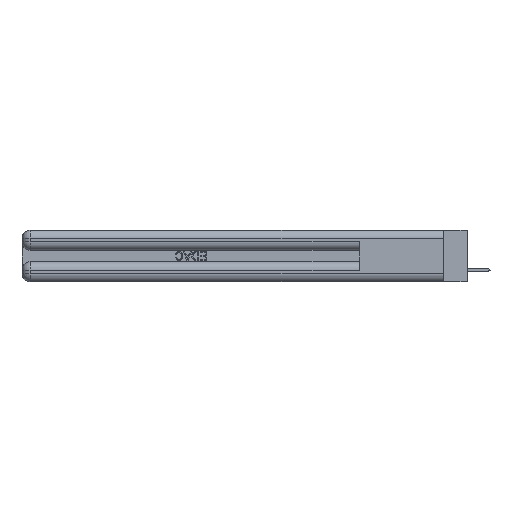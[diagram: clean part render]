
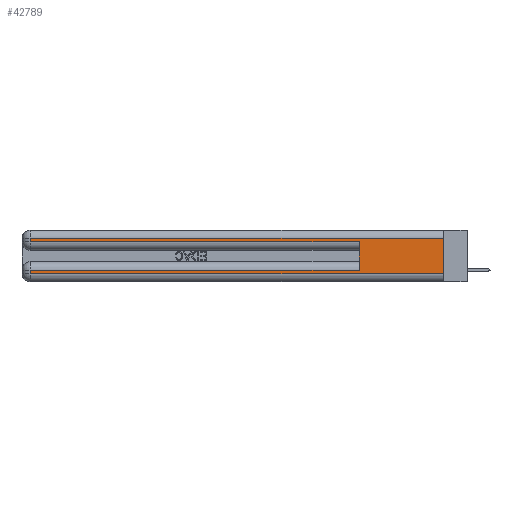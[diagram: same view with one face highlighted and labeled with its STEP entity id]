
A CAD part, left-side view. The second image highlights one B-rep face of the part: STEP entity #42789.
In plain terms, the highlighted planar face has unit normal (-1, 0, 0).
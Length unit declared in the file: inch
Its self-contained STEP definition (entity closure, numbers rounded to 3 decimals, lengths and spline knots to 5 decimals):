
#2408 = EDGE_CURVE ( 'NONE', #15796, #23937, #38843, .T. ) ;
#2837 = CARTESIAN_POINT ( 'NONE',  ( 0., 0., 0.31 ) ) ;
#3626 = DIRECTION ( 'NONE',  ( 0., 0., -1. ) ) ;
#3765 = LINE ( 'NONE', #13259, #15611 ) ;
#5084 = CARTESIAN_POINT ( 'NONE',  ( 0., 0., 0.285 ) ) ;
#5658 = LINE ( 'NONE', #5084, #23727 ) ;
#5894 = ORIENTED_EDGE ( 'NONE', *, *, #13150, .F. ) ;
#7551 = LINE ( 'NONE', #28737, #14400 ) ;
#7577 = LINE ( 'NONE', #15505, #40936 ) ;
#8554 = CARTESIAN_POINT ( 'NONE',  ( 0., 0., 0.085 ) ) ;
#9575 = ORIENTED_EDGE ( 'NONE', *, *, #38230, .T. ) ;
#9879 = EDGE_CURVE ( 'NONE', #10290, #16797, #5658, .T. ) ;
#10290 = VERTEX_POINT ( 'NONE', #37390 ) ;
#11018 = DIRECTION ( 'NONE',  ( 0., 1., 0. ) ) ;
#11537 = VECTOR ( 'NONE', #33886, 39.37008 ) ;
#12793 = CARTESIAN_POINT ( 'NONE',  ( 0., 0.6, 0.085 ) ) ;
#13150 = EDGE_CURVE ( 'NONE', #23504, #21130, #26059, .T. ) ;
#13259 = CARTESIAN_POINT ( 'NONE',  ( 0., 0., 0.06 ) ) ;
#14400 = VECTOR ( 'NONE', #11018, 39.37008 ) ;
#15348 = CARTESIAN_POINT ( 'NONE',  ( 0., 0., 0.37 ) ) ;
#15505 = CARTESIAN_POINT ( 'NONE',  ( 0., 0.6, 0.145 ) ) ;
#15611 = VECTOR ( 'NONE', #27459, 39.37008 ) ;
#15796 = VERTEX_POINT ( 'NONE', #34582 ) ;
#15822 = ORIENTED_EDGE ( 'NONE', *, *, #44929, .T. ) ;
#16546 = ORIENTED_EDGE ( 'NONE', *, *, #31710, .T. ) ;
#16797 = VERTEX_POINT ( 'NONE', #38414 ) ;
#17389 = CARTESIAN_POINT ( 'NONE',  ( 0., 2.94, 0.06 ) ) ;
#19365 = CARTESIAN_POINT ( 'NONE',  ( 0., 0., 0.37 ) ) ;
#19902 = EDGE_CURVE ( 'NONE', #32968, #16797, #7577, .T. ) ;
#20515 = AXIS2_PLACEMENT_3D ( 'NONE', #15348, #44396, #40641 ) ;
#20776 = VERTEX_POINT ( 'NONE', #32190 ) ;
#21130 = VERTEX_POINT ( 'NONE', #23594 ) ;
#21826 = VECTOR ( 'NONE', #3626, 39.37008 ) ;
#22173 = DIRECTION ( 'NONE',  ( 0., -1., 0. ) ) ;
#23504 = VERTEX_POINT ( 'NONE', #2837 ) ;
#23594 = CARTESIAN_POINT ( 'NONE',  ( 0., 0., 0.06 ) ) ;
#23727 = VECTOR ( 'NONE', #22173, 39.37008 ) ;
#23937 = VERTEX_POINT ( 'NONE', #17389 ) ;
#25581 = CARTESIAN_POINT ( 'NONE',  ( 0., 2.94, 0.37 ) ) ;
#26059 = LINE ( 'NONE', #19365, #28944 ) ;
#27459 = DIRECTION ( 'NONE',  ( 0., -1., 0. ) ) ;
#28737 = CARTESIAN_POINT ( 'NONE',  ( 0., 0., 0.31 ) ) ;
#28944 = VECTOR ( 'NONE', #34792, 39.37008 ) ;
#29761 = PLANE ( 'NONE',  #20515 ) ;
#31118 = FACE_OUTER_BOUND ( 'NONE', #32379, .T. ) ;
#31710 = EDGE_CURVE ( 'NONE', #23504, #20776, #7551, .T. ) ;
#32190 = CARTESIAN_POINT ( 'NONE',  ( 0., 2.94, 0.31 ) ) ;
#32365 = LINE ( 'NONE', #35673, #33428 ) ;
#32379 = EDGE_LOOP ( 'NONE', ( #5894, #16546, #15822, #42070, #40188, #36386, #36863, #9575 ) ) ;
#32525 = LINE ( 'NONE', #8554, #11537 ) ;
#32968 = VERTEX_POINT ( 'NONE', #12793 ) ;
#33428 = VECTOR ( 'NONE', #46225, 39.37008 ) ;
#33886 = DIRECTION ( 'NONE',  ( 0., 1., 0. ) ) ;
#34582 = CARTESIAN_POINT ( 'NONE',  ( 0., 2.94, 0.085 ) ) ;
#34792 = DIRECTION ( 'NONE',  ( 0., 0., -1. ) ) ;
#35673 = CARTESIAN_POINT ( 'NONE',  ( 0., 2.94, 0.37 ) ) ;
#36386 = ORIENTED_EDGE ( 'NONE', *, *, #39720, .T. ) ;
#36863 = ORIENTED_EDGE ( 'NONE', *, *, #2408, .T. ) ;
#37390 = CARTESIAN_POINT ( 'NONE',  ( 0., 2.94, 0.285 ) ) ;
#38230 = EDGE_CURVE ( 'NONE', #23937, #21130, #3765, .T. ) ;
#38414 = CARTESIAN_POINT ( 'NONE',  ( 0., 0.6, 0.285 ) ) ;
#38843 = LINE ( 'NONE', #25581, #21826 ) ;
#39720 = EDGE_CURVE ( 'NONE', #32968, #15796, #32525, .T. ) ;
#40188 = ORIENTED_EDGE ( 'NONE', *, *, #19902, .F. ) ;
#40641 = DIRECTION ( 'NONE',  ( 0., 0., -1. ) ) ;
#40936 = VECTOR ( 'NONE', #43709, 39.37008 ) ;
#42070 = ORIENTED_EDGE ( 'NONE', *, *, #9879, .T. ) ;
#42789 = ADVANCED_FACE ( 'NONE', ( #31118 ), #29761, .F. ) ;
#43709 = DIRECTION ( 'NONE',  ( 0., 0., 1. ) ) ;
#44396 = DIRECTION ( 'NONE',  ( 1., 0., 0. ) ) ;
#44929 = EDGE_CURVE ( 'NONE', #20776, #10290, #32365, .T. ) ;
#46225 = DIRECTION ( 'NONE',  ( 0., 0., -1. ) ) ;
